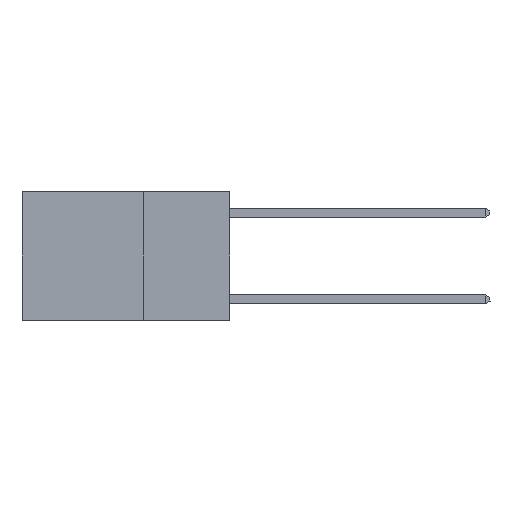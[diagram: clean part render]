
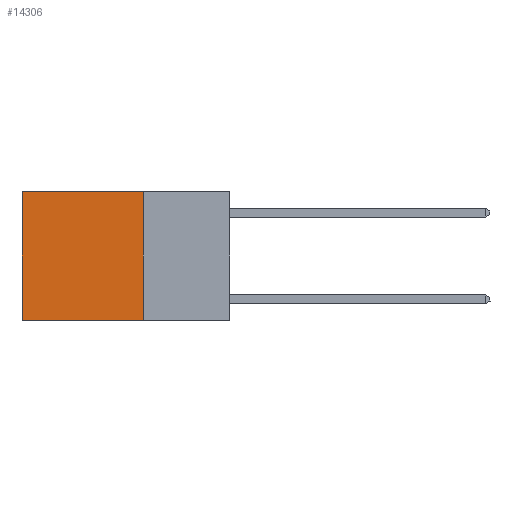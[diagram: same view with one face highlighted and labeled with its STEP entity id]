
A CAD part, left-side view. The second image highlights one B-rep face of the part: STEP entity #14306.
In plain terms, the highlighted planar face has unit normal (-1, 0, 0).
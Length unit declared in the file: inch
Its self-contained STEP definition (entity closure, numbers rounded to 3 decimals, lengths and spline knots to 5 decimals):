
#362 = VERTEX_POINT ( 'NONE', #14586 ) ;
#853 = CARTESIAN_POINT ( 'NONE',  ( 0.2625, 0.25, -0.37 ) ) ;
#945 = LINE ( 'NONE', #853, #8365 ) ;
#1504 = VECTOR ( 'NONE', #3301, 39.37008 ) ;
#1627 = ORIENTED_EDGE ( 'NONE', *, *, #12149, .F. ) ;
#3301 = DIRECTION ( 'NONE',  ( 0., 0., -1. ) ) ;
#5310 = DIRECTION ( 'NONE',  ( 1., 0., 0. ) ) ;
#5425 = LINE ( 'NONE', #7721, #1504 ) ;
#6360 = LINE ( 'NONE', #16361, #13804 ) ;
#7721 = CARTESIAN_POINT ( 'NONE',  ( 0.2625, 0.25, 0. ) ) ;
#8365 = VECTOR ( 'NONE', #12728, 39.37008 ) ;
#8542 = CARTESIAN_POINT ( 'NONE',  ( 0.2625, 0.6, -0.37 ) ) ;
#9378 = CARTESIAN_POINT ( 'NONE',  ( 0.2625, 0.25, 0. ) ) ;
#9719 = EDGE_CURVE ( 'NONE', #17125, #18135, #6360, .T. ) ;
#10850 = EDGE_LOOP ( 'NONE', ( #14565, #13146, #1627, #12771 ) ) ;
#11247 = PLANE ( 'NONE',  #14899 ) ;
#11978 = DIRECTION ( 'NONE',  ( 0., 1., 0. ) ) ;
#12124 = EDGE_CURVE ( 'NONE', #18135, #13035, #13813, .T. ) ;
#12149 = EDGE_CURVE ( 'NONE', #17125, #362, #5425, .T. ) ;
#12164 = CARTESIAN_POINT ( 'NONE',  ( 0.2625, 0.6, 0. ) ) ;
#12334 = FACE_OUTER_BOUND ( 'NONE', #10850, .T. ) ;
#12728 = DIRECTION ( 'NONE',  ( 0., 1., 0. ) ) ;
#12771 = ORIENTED_EDGE ( 'NONE', *, *, #9719, .T. ) ;
#13035 = VERTEX_POINT ( 'NONE', #8542 ) ;
#13146 = ORIENTED_EDGE ( 'NONE', *, *, #14305, .F. ) ;
#13804 = VECTOR ( 'NONE', #11978, 39.37008 ) ;
#13813 = LINE ( 'NONE', #12164, #17249 ) ;
#14219 = CARTESIAN_POINT ( 'NONE',  ( 0.2625, 0.25, 0. ) ) ;
#14305 = EDGE_CURVE ( 'NONE', #362, #13035, #945, .T. ) ;
#14306 = ADVANCED_FACE ( 'NONE', ( #12334 ), #11247, .F. ) ;
#14565 = ORIENTED_EDGE ( 'NONE', *, *, #12124, .T. ) ;
#14586 = CARTESIAN_POINT ( 'NONE',  ( 0.2625, 0.25, -0.37 ) ) ;
#14899 = AXIS2_PLACEMENT_3D ( 'NONE', #14219, #5310, #15697 ) ;
#15697 = DIRECTION ( 'NONE',  ( 0., 0., -1. ) ) ;
#16361 = CARTESIAN_POINT ( 'NONE',  ( 0.2625, 0.25, 0. ) ) ;
#17125 = VERTEX_POINT ( 'NONE', #9378 ) ;
#17249 = VECTOR ( 'NONE', #18054, 39.37008 ) ;
#18054 = DIRECTION ( 'NONE',  ( 0., 0., -1. ) ) ;
#18135 = VERTEX_POINT ( 'NONE', #18758 ) ;
#18758 = CARTESIAN_POINT ( 'NONE',  ( 0.2625, 0.6, 0. ) ) ;
